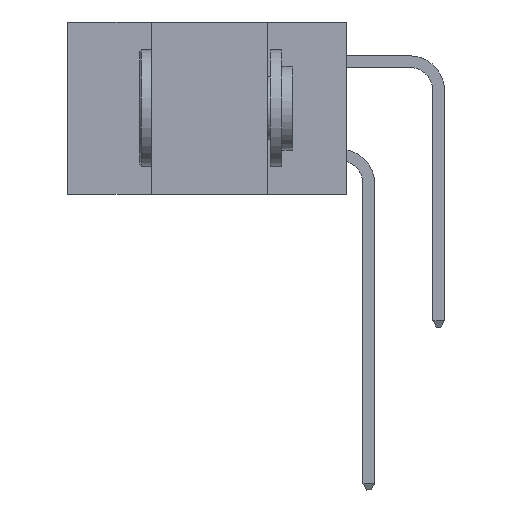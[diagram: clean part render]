
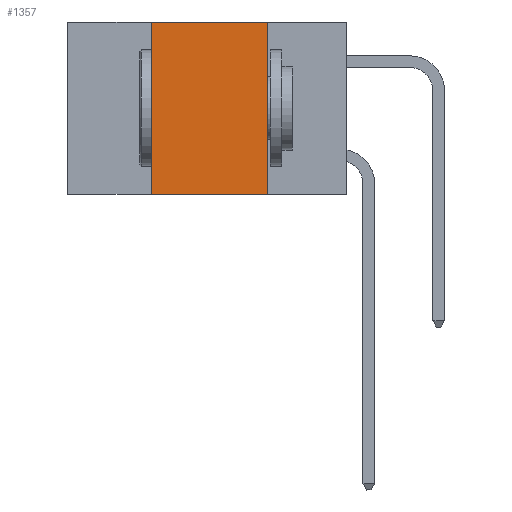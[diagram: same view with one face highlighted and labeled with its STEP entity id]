
A CAD part, left-side view. The second image highlights one B-rep face of the part: STEP entity #1357.
In plain terms, the highlighted planar face has unit normal (-1, 0, 0).
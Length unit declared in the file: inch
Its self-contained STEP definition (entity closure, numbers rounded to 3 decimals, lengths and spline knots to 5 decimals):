
#936 = DIRECTION ( 'NONE',  ( 0., -1., 0. ) ) ;
#1357 = ADVANCED_FACE ( 'NONE', ( #13425 ), #11764, .F. ) ;
#1466 = AXIS2_PLACEMENT_3D ( 'NONE', #9038, #9025, #9019 ) ;
#1535 = CARTESIAN_POINT ( 'NONE',  ( 0., 0.42, 0. ) ) ;
#1876 = VECTOR ( 'NONE', #7556, 39.37008 ) ;
#2662 = ORIENTED_EDGE ( 'NONE', *, *, #13875, .F. ) ;
#2715 = VERTEX_POINT ( 'NONE', #14051 ) ;
#3139 = EDGE_LOOP ( 'NONE', ( #2662, #13417, #14486, #5646 ) ) ;
#4193 = VERTEX_POINT ( 'NONE', #10505 ) ;
#4479 = CARTESIAN_POINT ( 'NONE',  ( 0., 0.6, 0. ) ) ;
#5058 = LINE ( 'NONE', #1535, #1876 ) ;
#5646 = ORIENTED_EDGE ( 'NONE', *, *, #6786, .T. ) ;
#6121 = VECTOR ( 'NONE', #936, 39.37008 ) ;
#6786 = EDGE_CURVE ( 'NONE', #8379, #14569, #8383, .T. ) ;
#7008 = CARTESIAN_POINT ( 'NONE',  ( 0., 0.6, -0.37 ) ) ;
#7556 = DIRECTION ( 'NONE',  ( 0., 0., 1. ) ) ;
#8256 = DIRECTION ( 'NONE',  ( 0., -1., 0. ) ) ;
#8379 = VERTEX_POINT ( 'NONE', #12256 ) ;
#8383 = LINE ( 'NONE', #7008, #11484 ) ;
#9019 = DIRECTION ( 'NONE',  ( 0., 0., -1. ) ) ;
#9025 = DIRECTION ( 'NONE',  ( 1., 0., 0. ) ) ;
#9038 = CARTESIAN_POINT ( 'NONE',  ( 0., 0.6, 0. ) ) ;
#9245 = VECTOR ( 'NONE', #13867, 39.37008 ) ;
#9612 = LINE ( 'NONE', #13817, #9245 ) ;
#10074 = EDGE_CURVE ( 'NONE', #8379, #4193, #5058, .T. ) ;
#10505 = CARTESIAN_POINT ( 'NONE',  ( 0., 0.42, 0. ) ) ;
#11395 = EDGE_CURVE ( 'NONE', #4193, #2715, #15079, .T. ) ;
#11484 = VECTOR ( 'NONE', #8256, 39.37008 ) ;
#11764 = PLANE ( 'NONE',  #1466 ) ;
#12256 = CARTESIAN_POINT ( 'NONE',  ( 0., 0.42, -0.37 ) ) ;
#12672 = CARTESIAN_POINT ( 'NONE',  ( 0., 0.17, -0.37 ) ) ;
#13417 = ORIENTED_EDGE ( 'NONE', *, *, #11395, .F. ) ;
#13425 = FACE_OUTER_BOUND ( 'NONE', #3139, .T. ) ;
#13817 = CARTESIAN_POINT ( 'NONE',  ( 0., 0.17, 0. ) ) ;
#13867 = DIRECTION ( 'NONE',  ( 0., 0., -1. ) ) ;
#13875 = EDGE_CURVE ( 'NONE', #2715, #14569, #9612, .T. ) ;
#14051 = CARTESIAN_POINT ( 'NONE',  ( 0., 0.17, 0. ) ) ;
#14486 = ORIENTED_EDGE ( 'NONE', *, *, #10074, .F. ) ;
#14569 = VERTEX_POINT ( 'NONE', #12672 ) ;
#15079 = LINE ( 'NONE', #4479, #6121 ) ;
